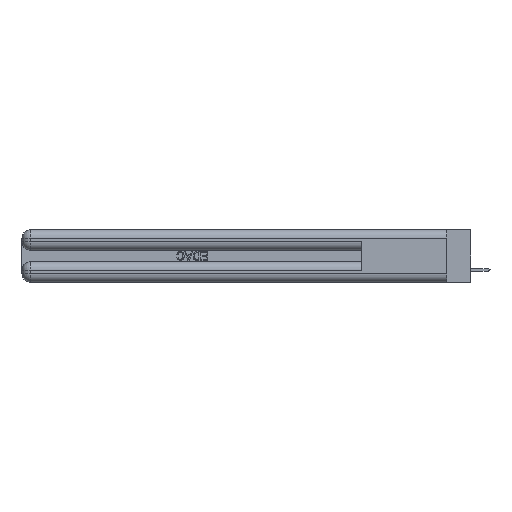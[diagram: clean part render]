
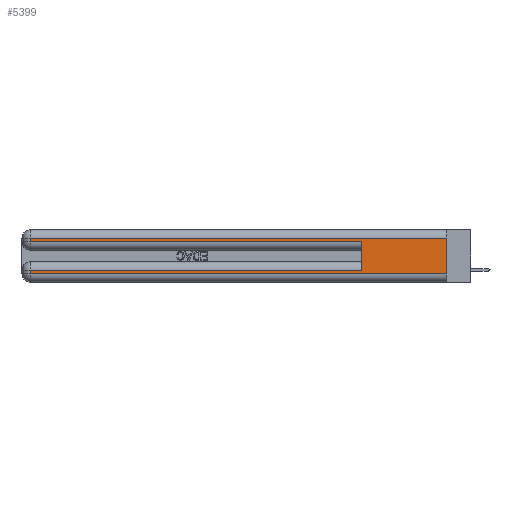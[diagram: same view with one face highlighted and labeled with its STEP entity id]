
A CAD part, left-side view. The second image highlights one B-rep face of the part: STEP entity #5399.
In plain terms, the highlighted planar face has unit normal (-1, 0, 0).
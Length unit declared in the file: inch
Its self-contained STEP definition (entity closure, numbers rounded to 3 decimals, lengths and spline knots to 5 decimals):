
#791 = LINE ( 'NONE', #20919, #14439 ) ;
#875 = DIRECTION ( 'NONE',  ( 0., 0., -1. ) ) ;
#1103 = VECTOR ( 'NONE', #14470, 39.37008 ) ;
#1246 = ORIENTED_EDGE ( 'NONE', *, *, #12506, .T. ) ;
#1304 = VECTOR ( 'NONE', #11301, 39.37008 ) ;
#1736 = LINE ( 'NONE', #4284, #24582 ) ;
#2380 = EDGE_CURVE ( 'NONE', #10548, #16703, #791, .T. ) ;
#2387 = VECTOR ( 'NONE', #34752, 39.37008 ) ;
#3233 = VERTEX_POINT ( 'NONE', #37979 ) ;
#3403 = CARTESIAN_POINT ( 'NONE',  ( 0., 0., 0.37 ) ) ;
#3429 = DIRECTION ( 'NONE',  ( 0., -1., 0. ) ) ;
#3652 = DIRECTION ( 'NONE',  ( 0., 0., -1. ) ) ;
#4239 = CARTESIAN_POINT ( 'NONE',  ( 0., 0., 0.31 ) ) ;
#4284 = CARTESIAN_POINT ( 'NONE',  ( 0., 2.94, 0.37 ) ) ;
#4788 = CARTESIAN_POINT ( 'NONE',  ( 0., 0., 0.085 ) ) ;
#5399 = ADVANCED_FACE ( 'NONE', ( #23929 ), #6750, .F. ) ;
#5906 = EDGE_CURVE ( 'NONE', #36246, #35647, #29863, .T. ) ;
#6372 = DIRECTION ( 'NONE',  ( 1., 0., 0. ) ) ;
#6750 = PLANE ( 'NONE',  #16333 ) ;
#8429 = CARTESIAN_POINT ( 'NONE',  ( 0., 0., 0.06 ) ) ;
#8536 = ORIENTED_EDGE ( 'NONE', *, *, #25491, .T. ) ;
#9399 = ORIENTED_EDGE ( 'NONE', *, *, #2380, .T. ) ;
#9615 = ORIENTED_EDGE ( 'NONE', *, *, #5906, .F. ) ;
#10248 = DIRECTION ( 'NONE',  ( 0., 0., -1. ) ) ;
#10548 = VERTEX_POINT ( 'NONE', #25818 ) ;
#11121 = EDGE_CURVE ( 'NONE', #3233, #17642, #28890, .T. ) ;
#11301 = DIRECTION ( 'NONE',  ( 0., -1., 0. ) ) ;
#11590 = LINE ( 'NONE', #17181, #1103 ) ;
#12310 = ORIENTED_EDGE ( 'NONE', *, *, #25499, .F. ) ;
#12506 = EDGE_CURVE ( 'NONE', #17642, #19767, #1736, .T. ) ;
#14087 = LINE ( 'NONE', #16976, #37531 ) ;
#14439 = VECTOR ( 'NONE', #32503, 39.37008 ) ;
#14470 = DIRECTION ( 'NONE',  ( 0., 0., 1. ) ) ;
#16333 = AXIS2_PLACEMENT_3D ( 'NONE', #18510, #6372, #3652 ) ;
#16703 = VERTEX_POINT ( 'NONE', #34052 ) ;
#16976 = CARTESIAN_POINT ( 'NONE',  ( 0., 0., 0.31 ) ) ;
#17181 = CARTESIAN_POINT ( 'NONE',  ( 0., 0.6, 0.145 ) ) ;
#17642 = VERTEX_POINT ( 'NONE', #28271 ) ;
#17680 = LINE ( 'NONE', #8429, #1304 ) ;
#18432 = CARTESIAN_POINT ( 'NONE',  ( 0., 2.94, 0.06 ) ) ;
#18510 = CARTESIAN_POINT ( 'NONE',  ( 0., 0., 0.37 ) ) ;
#18840 = CARTESIAN_POINT ( 'NONE',  ( 0., 0., 0.285 ) ) ;
#19451 = VERTEX_POINT ( 'NONE', #27751 ) ;
#19536 = ORIENTED_EDGE ( 'NONE', *, *, #20911, .T. ) ;
#19767 = VERTEX_POINT ( 'NONE', #18432 ) ;
#20911 = EDGE_CURVE ( 'NONE', #16703, #19451, #29689, .T. ) ;
#20919 = CARTESIAN_POINT ( 'NONE',  ( 0., 2.94, 0.37 ) ) ;
#21869 = VECTOR ( 'NONE', #875, 39.37008 ) ;
#23929 = FACE_OUTER_BOUND ( 'NONE', #24025, .T. ) ;
#24025 = EDGE_LOOP ( 'NONE', ( #9615, #8536, #9399, #19536, #12310, #29226, #1246, #33807 ) ) ;
#24582 = VECTOR ( 'NONE', #10248, 39.37008 ) ;
#25491 = EDGE_CURVE ( 'NONE', #36246, #10548, #14087, .T. ) ;
#25499 = EDGE_CURVE ( 'NONE', #3233, #19451, #11590, .T. ) ;
#25818 = CARTESIAN_POINT ( 'NONE',  ( 0., 2.94, 0.31 ) ) ;
#25878 = DIRECTION ( 'NONE',  ( 0., 1., 0. ) ) ;
#27751 = CARTESIAN_POINT ( 'NONE',  ( 0., 0.6, 0.285 ) ) ;
#28271 = CARTESIAN_POINT ( 'NONE',  ( 0., 2.94, 0.085 ) ) ;
#28890 = LINE ( 'NONE', #4788, #2387 ) ;
#29226 = ORIENTED_EDGE ( 'NONE', *, *, #11121, .T. ) ;
#29689 = LINE ( 'NONE', #18840, #33050 ) ;
#29863 = LINE ( 'NONE', #3403, #21869 ) ;
#31676 = EDGE_CURVE ( 'NONE', #19767, #35647, #17680, .T. ) ;
#32503 = DIRECTION ( 'NONE',  ( 0., 0., -1. ) ) ;
#33050 = VECTOR ( 'NONE', #3429, 39.37008 ) ;
#33767 = CARTESIAN_POINT ( 'NONE',  ( 0., 0., 0.06 ) ) ;
#33807 = ORIENTED_EDGE ( 'NONE', *, *, #31676, .T. ) ;
#34052 = CARTESIAN_POINT ( 'NONE',  ( 0., 2.94, 0.285 ) ) ;
#34752 = DIRECTION ( 'NONE',  ( 0., 1., 0. ) ) ;
#35647 = VERTEX_POINT ( 'NONE', #33767 ) ;
#36246 = VERTEX_POINT ( 'NONE', #4239 ) ;
#37531 = VECTOR ( 'NONE', #25878, 39.37008 ) ;
#37979 = CARTESIAN_POINT ( 'NONE',  ( 0., 0.6, 0.085 ) ) ;
